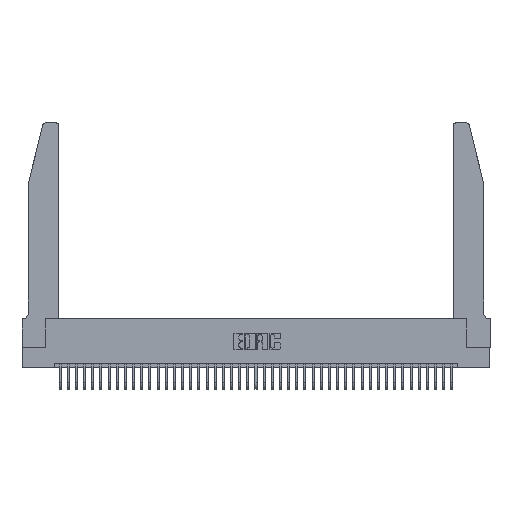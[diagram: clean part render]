
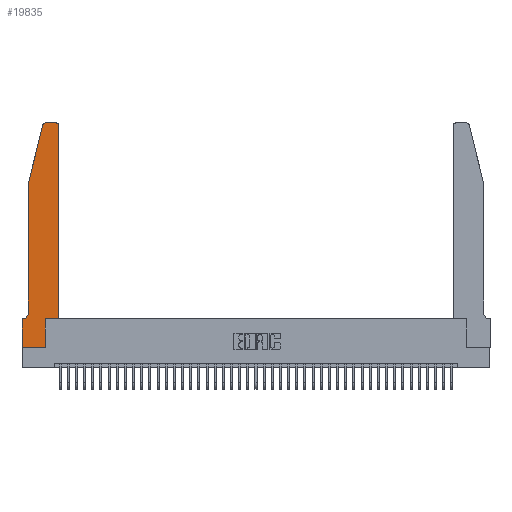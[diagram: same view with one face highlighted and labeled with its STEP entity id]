
A CAD part, top view. The second image highlights one B-rep face of the part: STEP entity #19835.
In plain terms, the highlighted planar face has unit normal (0, 0, 1).
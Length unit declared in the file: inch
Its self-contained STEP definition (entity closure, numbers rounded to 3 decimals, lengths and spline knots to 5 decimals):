
#326 = VERTEX_POINT ( 'NONE', #9200 ) ;
#789 = AXIS2_PLACEMENT_3D ( 'NONE', #4344, #26397, #7522 ) ;
#1194 = EDGE_CURVE ( 'NONE', #4024, #22616, #30218, .T. ) ;
#1449 = DIRECTION ( 'NONE',  ( 0., 0., 1. ) ) ;
#2526 = ORIENTED_EDGE ( 'NONE', *, *, #14396, .T. ) ;
#2649 = EDGE_CURVE ( 'NONE', #34802, #13333, #9917, .T. ) ;
#3713 = VERTEX_POINT ( 'NONE', #35669 ) ;
#3989 = LINE ( 'NONE', #30155, #4973 ) ;
#4024 = VERTEX_POINT ( 'NONE', #34296 ) ;
#4344 = CARTESIAN_POINT ( 'NONE',  ( 0.0055, 0.42, 0.37 ) ) ;
#4967 = VERTEX_POINT ( 'NONE', #39828 ) ;
#4973 = VECTOR ( 'NONE', #11278, 39.37008 ) ;
#5372 = CARTESIAN_POINT ( 'NONE',  ( 0.4505, 2.72, 0.37 ) ) ;
#5502 = LINE ( 'NONE', #32662, #29646 ) ;
#7198 = DIRECTION ( 'NONE',  ( 1., 0., 0. ) ) ;
#7522 = DIRECTION ( 'NONE',  ( -1., 0., 0. ) ) ;
#8377 = CARTESIAN_POINT ( 'NONE',  ( 0.2865, 0., 0.37 ) ) ;
#8424 = DIRECTION ( 'NONE',  ( 0., -1., 0. ) ) ;
#8473 = LINE ( 'NONE', #16403, #16823 ) ;
#8830 = LINE ( 'NONE', #34602, #25613 ) ;
#8927 = EDGE_CURVE ( 'NONE', #21244, #38646, #8830, .T. ) ;
#9200 = CARTESIAN_POINT ( 'NONE',  ( 0.25487, 2.72718, 0.37 ) ) ;
#9434 = DIRECTION ( 'NONE',  ( 0., -1., 0. ) ) ;
#9917 = CIRCLE ( 'NONE', #38078, 0.03 ) ;
#10314 = VECTOR ( 'NONE', #16163, 39.37008 ) ;
#11278 = DIRECTION ( 'NONE',  ( 0., 1., 0. ) ) ;
#11900 = EDGE_CURVE ( 'NONE', #3713, #4024, #40112, .T. ) ;
#13333 = VERTEX_POINT ( 'NONE', #28035 ) ;
#13579 = VECTOR ( 'NONE', #34480, 39.37008 ) ;
#13772 = DIRECTION ( 'NONE',  ( -1., 0., 0. ) ) ;
#14031 = VECTOR ( 'NONE', #8424, 39.37008 ) ;
#14035 = CARTESIAN_POINT ( 'NONE',  ( 0.284, 2.72, 0.37 ) ) ;
#14148 = VERTEX_POINT ( 'NONE', #16104 ) ;
#14396 = EDGE_CURVE ( 'NONE', #22616, #29672, #3989, .T. ) ;
#14428 = VECTOR ( 'NONE', #16274, 39.37008 ) ;
#15570 = DIRECTION ( 'NONE',  ( 0., 0., 1. ) ) ;
#16104 = CARTESIAN_POINT ( 'NONE',  ( 0.284, 2.75, 0.37 ) ) ;
#16163 = DIRECTION ( 'NONE',  ( 0., 1., 0. ) ) ;
#16274 = DIRECTION ( 'NONE',  ( 1., 0., 0. ) ) ;
#16403 = CARTESIAN_POINT ( 'NONE',  ( 0.0755, 2., 0.37 ) ) ;
#16536 = VERTEX_POINT ( 'NONE', #25333 ) ;
#16823 = VECTOR ( 'NONE', #35259, 39.37008 ) ;
#17137 = LINE ( 'NONE', #38506, #24592 ) ;
#17182 = DIRECTION ( 'NONE',  ( 1., 0., 0. ) ) ;
#18128 = EDGE_CURVE ( 'NONE', #13333, #14148, #5502, .T. ) ;
#18831 = ORIENTED_EDGE ( 'NONE', *, *, #1194, .T. ) ;
#19268 = EDGE_CURVE ( 'NONE', #16536, #34802, #19657, .T. ) ;
#19657 = LINE ( 'NONE', #31894, #10314 ) ;
#19835 = ADVANCED_FACE ( 'NONE', ( #31461 ), #31300, .T. ) ;
#19954 = ORIENTED_EDGE ( 'NONE', *, *, #11900, .T. ) ;
#20311 = CARTESIAN_POINT ( 'NONE',  ( 0.4205, 2.72, 0.37 ) ) ;
#20568 = ORIENTED_EDGE ( 'NONE', *, *, #18128, .T. ) ;
#20717 = CIRCLE ( 'NONE', #789, 0.07 ) ;
#21244 = VERTEX_POINT ( 'NONE', #26271 ) ;
#21819 = EDGE_CURVE ( 'NONE', #326, #21244, #8473, .T. ) ;
#22616 = VERTEX_POINT ( 'NONE', #8377 ) ;
#22899 = ORIENTED_EDGE ( 'NONE', *, *, #2649, .T. ) ;
#23467 = DIRECTION ( 'NONE',  ( 1., 0., 0. ) ) ;
#24592 = VECTOR ( 'NONE', #7198, 39.37008 ) ;
#24719 = CARTESIAN_POINT ( 'NONE',  ( 0.2865, 0.35, 0.37 ) ) ;
#24911 = CIRCLE ( 'NONE', #26340, 0.03 ) ;
#25166 = ORIENTED_EDGE ( 'NONE', *, *, #25796, .T. ) ;
#25333 = CARTESIAN_POINT ( 'NONE',  ( 0.4505, 0.35, 0.37 ) ) ;
#25613 = VECTOR ( 'NONE', #9434, 39.37008 ) ;
#25796 = EDGE_CURVE ( 'NONE', #4967, #3713, #38647, .T. ) ;
#26271 = CARTESIAN_POINT ( 'NONE',  ( 0.0755, 2., 0.37 ) ) ;
#26340 = AXIS2_PLACEMENT_3D ( 'NONE', #14035, #36035, #17182 ) ;
#26397 = DIRECTION ( 'NONE',  ( 0., 0., -1. ) ) ;
#28033 = ORIENTED_EDGE ( 'NONE', *, *, #19268, .T. ) ;
#28035 = CARTESIAN_POINT ( 'NONE',  ( 0.4205, 2.75, 0.37 ) ) ;
#29646 = VECTOR ( 'NONE', #13772, 39.37008 ) ;
#29672 = VERTEX_POINT ( 'NONE', #24719 ) ;
#30155 = CARTESIAN_POINT ( 'NONE',  ( 0.2865, 0.35, 0.37 ) ) ;
#30218 = LINE ( 'NONE', #35132, #14428 ) ;
#31300 = PLANE ( 'NONE',  #36511 ) ;
#31357 = CARTESIAN_POINT ( 'NONE',  ( 0.0755, 0.35, 0.37 ) ) ;
#31461 = FACE_OUTER_BOUND ( 'NONE', #40047, .T. ) ;
#31894 = CARTESIAN_POINT ( 'NONE',  ( 0.4505, 0.35, 0.37 ) ) ;
#32261 = ORIENTED_EDGE ( 'NONE', *, *, #39981, .T. ) ;
#32662 = CARTESIAN_POINT ( 'NONE',  ( 0.2605, 2.75, 0.37 ) ) ;
#34296 = CARTESIAN_POINT ( 'NONE',  ( 0., 0., 0.37 ) ) ;
#34381 = ORIENTED_EDGE ( 'NONE', *, *, #34531, .T. ) ;
#34431 = CARTESIAN_POINT ( 'NONE',  ( 0., 0.35, 0.37 ) ) ;
#34480 = DIRECTION ( 'NONE',  ( -1., 0., 0. ) ) ;
#34531 = EDGE_CURVE ( 'NONE', #29672, #16536, #17137, .T. ) ;
#34602 = CARTESIAN_POINT ( 'NONE',  ( 0.0755, 2., 0.37 ) ) ;
#34802 = VERTEX_POINT ( 'NONE', #5372 ) ;
#35132 = CARTESIAN_POINT ( 'NONE',  ( 0., 0., 0.37 ) ) ;
#35259 = DIRECTION ( 'NONE',  ( -0.239, -0.971, 0. ) ) ;
#35384 = CARTESIAN_POINT ( 'NONE',  ( 0.0755, 0.42, 0.37 ) ) ;
#35669 = CARTESIAN_POINT ( 'NONE',  ( 0., 0.35, 0.37 ) ) ;
#35878 = ORIENTED_EDGE ( 'NONE', *, *, #21819, .T. ) ;
#36035 = DIRECTION ( 'NONE',  ( 0., 0., 1. ) ) ;
#36497 = EDGE_CURVE ( 'NONE', #14148, #326, #24911, .T. ) ;
#36511 = AXIS2_PLACEMENT_3D ( 'NONE', #34431, #15570, #37567 ) ;
#36614 = CARTESIAN_POINT ( 'NONE',  ( 0., 0., 0.37 ) ) ;
#37567 = DIRECTION ( 'NONE',  ( 1., 0., 0. ) ) ;
#38078 = AXIS2_PLACEMENT_3D ( 'NONE', #20311, #1449, #23467 ) ;
#38449 = ORIENTED_EDGE ( 'NONE', *, *, #36497, .T. ) ;
#38506 = CARTESIAN_POINT ( 'NONE',  ( 0.4505, 0.35, 0.37 ) ) ;
#38646 = VERTEX_POINT ( 'NONE', #35384 ) ;
#38647 = LINE ( 'NONE', #31357, #13579 ) ;
#39828 = CARTESIAN_POINT ( 'NONE',  ( 0.0055, 0.35, 0.37 ) ) ;
#39981 = EDGE_CURVE ( 'NONE', #38646, #4967, #20717, .T. ) ;
#40047 = EDGE_LOOP ( 'NONE', ( #20568, #38449, #35878, #40303, #32261, #25166, #19954, #18831, #2526, #34381, #28033, #22899 ) ) ;
#40112 = LINE ( 'NONE', #36614, #14031 ) ;
#40303 = ORIENTED_EDGE ( 'NONE', *, *, #8927, .T. ) ;
